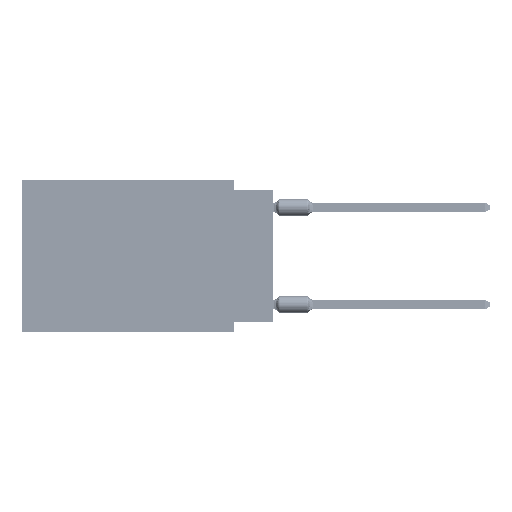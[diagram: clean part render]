
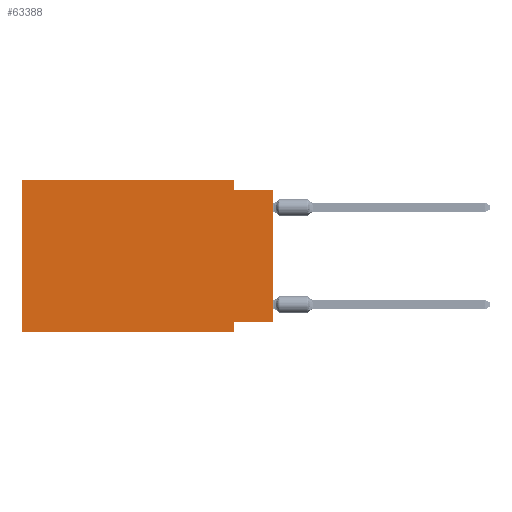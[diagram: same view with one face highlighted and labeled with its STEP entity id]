
A CAD part, left-side view. The second image highlights one B-rep face of the part: STEP entity #63388.
In plain terms, the highlighted planar face has unit normal (-1, 0, 0).
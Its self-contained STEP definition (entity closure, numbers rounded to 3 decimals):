
#178 = VECTOR ( 'NONE', #72444, 1000. ) ;
#4240 = CARTESIAN_POINT ( 'NONE',  ( 0., 16.383, 0. ) ) ;
#4836 = LINE ( 'NONE', #67441, #72211 ) ;
#5281 = VERTEX_POINT ( 'NONE', #42194 ) ;
#6290 = ORIENTED_EDGE ( 'NONE', *, *, #40869, .F. ) ;
#6531 = VERTEX_POINT ( 'NONE', #69299 ) ;
#6555 = CARTESIAN_POINT ( 'NONE',  ( 0., 2.54, -9.906 ) ) ;
#8116 = CARTESIAN_POINT ( 'NONE',  ( 0., 0., -9.271 ) ) ;
#8319 = VERTEX_POINT ( 'NONE', #49511 ) ;
#8448 = VECTOR ( 'NONE', #41227, 1000. ) ;
#9310 = LINE ( 'NONE', #65256, #26646 ) ;
#10520 = DIRECTION ( 'NONE',  ( 0., 0., -1. ) ) ;
#10695 = DIRECTION ( 'NONE',  ( 0., 0., 1. ) ) ;
#10909 = ORIENTED_EDGE ( 'NONE', *, *, #43772, .T. ) ;
#11624 = EDGE_CURVE ( 'NONE', #20631, #37941, #30207, .T. ) ;
#12474 = DIRECTION ( 'NONE',  ( 0., 0., -1. ) ) ;
#16480 = CARTESIAN_POINT ( 'NONE',  ( 0., 16.383, 0. ) ) ;
#20038 = DIRECTION ( 'NONE',  ( 0., -1., 0. ) ) ;
#20395 = ORIENTED_EDGE ( 'NONE', *, *, #66030, .F. ) ;
#20631 = VERTEX_POINT ( 'NONE', #8116 ) ;
#20827 = VECTOR ( 'NONE', #12474, 1000. ) ;
#21535 = VECTOR ( 'NONE', #10695, 1000. ) ;
#24649 = CARTESIAN_POINT ( 'NONE',  ( 0., 0., 0. ) ) ;
#25459 = DIRECTION ( 'NONE',  ( 0., -1., 0. ) ) ;
#26137 = ORIENTED_EDGE ( 'NONE', *, *, #48186, .F. ) ;
#26455 = DIRECTION ( 'NONE',  ( 1., 0., 0. ) ) ;
#26646 = VECTOR ( 'NONE', #20038, 1000. ) ;
#27782 = VERTEX_POINT ( 'NONE', #68395 ) ;
#28794 = CARTESIAN_POINT ( 'NONE',  ( 0., 16.383, 0. ) ) ;
#28975 = AXIS2_PLACEMENT_3D ( 'NONE', #4240, #26455, #10520 ) ;
#30207 = LINE ( 'NONE', #24649, #55862 ) ;
#33084 = ORIENTED_EDGE ( 'NONE', *, *, #11624, .T. ) ;
#36550 = LINE ( 'NONE', #70287, #58395 ) ;
#37569 = PLANE ( 'NONE',  #28975 ) ;
#37941 = VERTEX_POINT ( 'NONE', #71718 ) ;
#40401 = CARTESIAN_POINT ( 'NONE',  ( 0., 16.383, -9.906 ) ) ;
#40869 = EDGE_CURVE ( 'NONE', #8319, #27782, #64228, .T. ) ;
#41227 = DIRECTION ( 'NONE',  ( 0., 0., -1. ) ) ;
#42194 = CARTESIAN_POINT ( 'NONE',  ( 0., 2.54, -9.906 ) ) ;
#43510 = DIRECTION ( 'NONE',  ( 0., 0., 1. ) ) ;
#43772 = EDGE_CURVE ( 'NONE', #71495, #5281, #9310, .T. ) ;
#46151 = LINE ( 'NONE', #6555, #20827 ) ;
#48186 = EDGE_CURVE ( 'NONE', #71495, #65602, #72187, .T. ) ;
#49511 = CARTESIAN_POINT ( 'NONE',  ( 0., 2.54, 0. ) ) ;
#49726 = EDGE_CURVE ( 'NONE', #27782, #37941, #36550, .T. ) ;
#49805 = LINE ( 'NONE', #16480, #178 ) ;
#55212 = DIRECTION ( 'NONE',  ( 0., 1., 0. ) ) ;
#55862 = VECTOR ( 'NONE', #43510, 1000. ) ;
#58395 = VECTOR ( 'NONE', #25459, 1000. ) ;
#60123 = ORIENTED_EDGE ( 'NONE', *, *, #64470, .F. ) ;
#63388 = ADVANCED_FACE ( 'NONE', ( #72383 ), #37569, .F. ) ;
#63926 = ORIENTED_EDGE ( 'NONE', *, *, #49726, .F. ) ;
#64228 = LINE ( 'NONE', #69759, #8448 ) ;
#64470 = EDGE_CURVE ( 'NONE', #6531, #5281, #46151, .T. ) ;
#65256 = CARTESIAN_POINT ( 'NONE',  ( 0., 16.383, -9.906 ) ) ;
#65602 = VERTEX_POINT ( 'NONE', #28794 ) ;
#66030 = EDGE_CURVE ( 'NONE', #65602, #8319, #49805, .T. ) ;
#66655 = CARTESIAN_POINT ( 'NONE',  ( 0., 16.383, 0. ) ) ;
#66688 = ORIENTED_EDGE ( 'NONE', *, *, #66921, .F. ) ;
#66797 = EDGE_LOOP ( 'NONE', ( #33084, #63926, #6290, #20395, #26137, #10909, #60123, #66688 ) ) ;
#66921 = EDGE_CURVE ( 'NONE', #20631, #6531, #4836, .T. ) ;
#67441 = CARTESIAN_POINT ( 'NONE',  ( 0., 0., -9.271 ) ) ;
#68395 = CARTESIAN_POINT ( 'NONE',  ( 0., 2.54, -0.635 ) ) ;
#69299 = CARTESIAN_POINT ( 'NONE',  ( 0., 2.54, -9.271 ) ) ;
#69759 = CARTESIAN_POINT ( 'NONE',  ( 0., 2.54, 0. ) ) ;
#70287 = CARTESIAN_POINT ( 'NONE',  ( 0., 0., -0.635 ) ) ;
#71495 = VERTEX_POINT ( 'NONE', #40401 ) ;
#71718 = CARTESIAN_POINT ( 'NONE',  ( 0., 0., -0.635 ) ) ;
#72187 = LINE ( 'NONE', #66655, #21535 ) ;
#72211 = VECTOR ( 'NONE', #55212, 1000. ) ;
#72383 = FACE_OUTER_BOUND ( 'NONE', #66797, .T. ) ;
#72444 = DIRECTION ( 'NONE',  ( 0., -1., 0. ) ) ;
